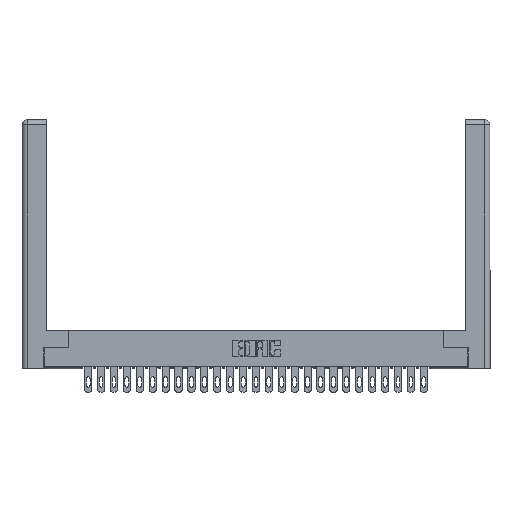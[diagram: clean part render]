
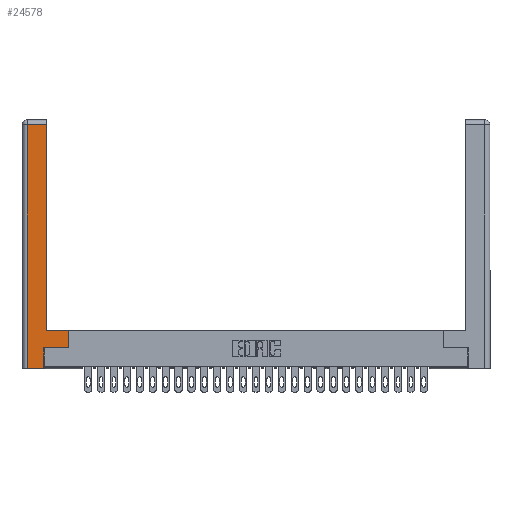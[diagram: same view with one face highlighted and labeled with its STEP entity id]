
A CAD part, top view. The second image highlights one B-rep face of the part: STEP entity #24578.
In plain terms, the highlighted planar face has unit normal (0, 0, 1).
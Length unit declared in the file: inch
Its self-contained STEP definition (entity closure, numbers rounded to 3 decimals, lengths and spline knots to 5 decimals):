
#706 = LINE ( 'NONE', #29236, #13814 ) ;
#871 = VERTEX_POINT ( 'NONE', #26355 ) ;
#947 = CARTESIAN_POINT ( 'NONE',  ( 0.565, 0.45, 0. ) ) ;
#1704 = DIRECTION ( 'NONE',  ( -1., 0., 0. ) ) ;
#2219 = VECTOR ( 'NONE', #19557, 39.37008 ) ;
#2913 = VECTOR ( 'NONE', #12347, 39.37008 ) ;
#2924 = ORIENTED_EDGE ( 'NONE', *, *, #15772, .T. ) ;
#3266 = CARTESIAN_POINT ( 'NONE',  ( 0.295, 3., 0. ) ) ;
#4164 = LINE ( 'NONE', #11744, #21324 ) ;
#4574 = LINE ( 'NONE', #26748, #27746 ) ;
#5146 = AXIS2_PLACEMENT_3D ( 'NONE', #17466, #28997, #15285 ) ;
#5827 = VECTOR ( 'NONE', #15555, 39.37008 ) ;
#6277 = ORIENTED_EDGE ( 'NONE', *, *, #18814, .T. ) ;
#6348 = CARTESIAN_POINT ( 'NONE',  ( 0.0615, 2.94, 0. ) ) ;
#6724 = CARTESIAN_POINT ( 'NONE',  ( 0.295, 0.45, 0. ) ) ;
#8952 = LINE ( 'NONE', #28135, #20570 ) ;
#9213 = CARTESIAN_POINT ( 'NONE',  ( 0.565, 0.245, 0. ) ) ;
#9508 = CARTESIAN_POINT ( 'NONE',  ( 0.295, 0.45, 0. ) ) ;
#10852 = CARTESIAN_POINT ( 'NONE',  ( 0.0615, 0., 0. ) ) ;
#11014 = ORIENTED_EDGE ( 'NONE', *, *, #17370, .T. ) ;
#11637 = LINE ( 'NONE', #10852, #5827 ) ;
#11744 = CARTESIAN_POINT ( 'NONE',  ( 0.565, 0.245, 0. ) ) ;
#12160 = EDGE_CURVE ( 'NONE', #12720, #24102, #706, .T. ) ;
#12347 = DIRECTION ( 'NONE',  ( -1., 0., 0. ) ) ;
#12720 = VERTEX_POINT ( 'NONE', #13240 ) ;
#12953 = DIRECTION ( 'NONE',  ( 0., 1., 0. ) ) ;
#13240 = CARTESIAN_POINT ( 'NONE',  ( 0.0615, 0., 0. ) ) ;
#13557 = VERTEX_POINT ( 'NONE', #9213 ) ;
#13814 = VECTOR ( 'NONE', #15521, 39.37008 ) ;
#13886 = EDGE_CURVE ( 'NONE', #24102, #15572, #4574, .T. ) ;
#14095 = DIRECTION ( 'NONE',  ( 1., 0., 0. ) ) ;
#15078 = ORIENTED_EDGE ( 'NONE', *, *, #12160, .T. ) ;
#15187 = ORIENTED_EDGE ( 'NONE', *, *, #21549, .T. ) ;
#15285 = DIRECTION ( 'NONE',  ( -1., 0., 0. ) ) ;
#15521 = DIRECTION ( 'NONE',  ( 1., 0., 0. ) ) ;
#15555 = DIRECTION ( 'NONE',  ( 0., -1., 0. ) ) ;
#15572 = VERTEX_POINT ( 'NONE', #21821 ) ;
#15772 = EDGE_CURVE ( 'NONE', #871, #24874, #18686, .T. ) ;
#16396 = VERTEX_POINT ( 'NONE', #6724 ) ;
#17321 = EDGE_CURVE ( 'NONE', #27825, #16396, #28241, .T. ) ;
#17356 = ORIENTED_EDGE ( 'NONE', *, *, #25606, .T. ) ;
#17370 = EDGE_CURVE ( 'NONE', #16396, #871, #26111, .T. ) ;
#17466 = CARTESIAN_POINT ( 'NONE',  ( 0., 0., 0. ) ) ;
#17964 = VECTOR ( 'NONE', #1704, 39.37008 ) ;
#18686 = LINE ( 'NONE', #6348, #17964 ) ;
#18814 = EDGE_CURVE ( 'NONE', #24874, #12720, #11637, .T. ) ;
#19557 = DIRECTION ( 'NONE',  ( 0., 1., 0. ) ) ;
#19827 = ORIENTED_EDGE ( 'NONE', *, *, #17321, .T. ) ;
#20281 = FACE_OUTER_BOUND ( 'NONE', #23715, .T. ) ;
#20570 = VECTOR ( 'NONE', #25860, 39.37008 ) ;
#20902 = CARTESIAN_POINT ( 'NONE',  ( 0.0615, 2.94, 0. ) ) ;
#21324 = VECTOR ( 'NONE', #14095, 39.37008 ) ;
#21549 = EDGE_CURVE ( 'NONE', #15572, #13557, #4164, .T. ) ;
#21821 = CARTESIAN_POINT ( 'NONE',  ( 0.265, 0.245, 0. ) ) ;
#22138 = PLANE ( 'NONE',  #5146 ) ;
#22759 = CARTESIAN_POINT ( 'NONE',  ( 0.265, 0., 0. ) ) ;
#23715 = EDGE_LOOP ( 'NONE', ( #11014, #2924, #6277, #15078, #26650, #15187, #17356, #19827 ) ) ;
#24102 = VERTEX_POINT ( 'NONE', #22759 ) ;
#24578 = ADVANCED_FACE ( 'NONE', ( #20281 ), #22138, .F. ) ;
#24874 = VERTEX_POINT ( 'NONE', #20902 ) ;
#25606 = EDGE_CURVE ( 'NONE', #13557, #27825, #8952, .T. ) ;
#25860 = DIRECTION ( 'NONE',  ( 0., 1., 0. ) ) ;
#26111 = LINE ( 'NONE', #3266, #2219 ) ;
#26355 = CARTESIAN_POINT ( 'NONE',  ( 0.295, 2.94, 0. ) ) ;
#26650 = ORIENTED_EDGE ( 'NONE', *, *, #13886, .T. ) ;
#26748 = CARTESIAN_POINT ( 'NONE',  ( 0.265, 0.245, 0. ) ) ;
#27746 = VECTOR ( 'NONE', #12953, 39.37008 ) ;
#27825 = VERTEX_POINT ( 'NONE', #947 ) ;
#28135 = CARTESIAN_POINT ( 'NONE',  ( 0.565, 0.45, 0. ) ) ;
#28241 = LINE ( 'NONE', #9508, #2913 ) ;
#28997 = DIRECTION ( 'NONE',  ( 0., 0., -1. ) ) ;
#29236 = CARTESIAN_POINT ( 'NONE',  ( 0.265, 0., 0. ) ) ;
